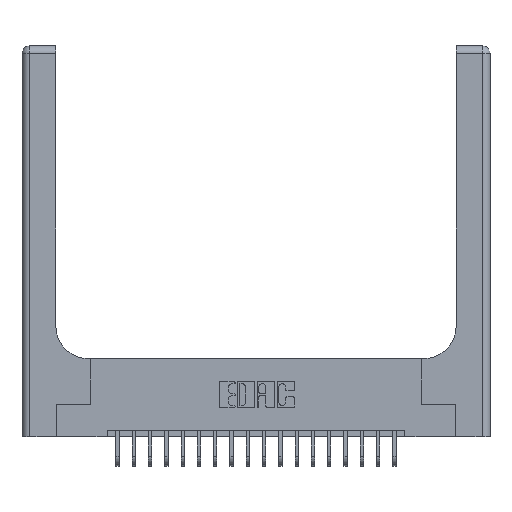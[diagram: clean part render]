
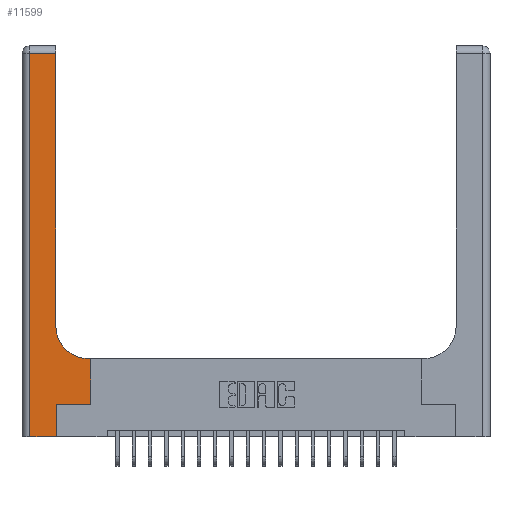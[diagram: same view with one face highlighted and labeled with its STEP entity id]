
A CAD part, top view. The second image highlights one B-rep face of the part: STEP entity #11599.
In plain terms, the highlighted planar face has unit normal (0, 0, 1).
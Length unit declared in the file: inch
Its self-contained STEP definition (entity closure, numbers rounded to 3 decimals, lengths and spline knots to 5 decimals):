
#209 = DIRECTION ( 'NONE',  ( 1., 0., 0. ) ) ;
#285 = CARTESIAN_POINT ( 'NONE',  ( 0.26, 2.94, 0.37 ) ) ;
#312 = LINE ( 'NONE', #4425, #4010 ) ;
#633 = VERTEX_POINT ( 'NONE', #685 ) ;
#685 = CARTESIAN_POINT ( 'NONE',  ( 0.51, 0.6, 0.37 ) ) ;
#1783 = DIRECTION ( 'NONE',  ( -1., 0., 0. ) ) ;
#2127 = VERTEX_POINT ( 'NONE', #19964 ) ;
#2364 = ORIENTED_EDGE ( 'NONE', *, *, #2592, .T. ) ;
#2566 = CARTESIAN_POINT ( 'NONE',  ( 0.06, 2.94, 0.37 ) ) ;
#2592 = EDGE_CURVE ( 'NONE', #12691, #8772, #11009, .T. ) ;
#2869 = CARTESIAN_POINT ( 'NONE',  ( 0.265, 0., 0.37 ) ) ;
#3447 = DIRECTION ( 'NONE',  ( 0., 1., 0. ) ) ;
#3495 = LINE ( 'NONE', #10424, #6220 ) ;
#3815 = ORIENTED_EDGE ( 'NONE', *, *, #8806, .T. ) ;
#4010 = VECTOR ( 'NONE', #4310, 39.37008 ) ;
#4310 = DIRECTION ( 'NONE',  ( 1., 0., 0. ) ) ;
#4425 = CARTESIAN_POINT ( 'NONE',  ( 0.265, 0.25, 0.37 ) ) ;
#4472 = LINE ( 'NONE', #2869, #11944 ) ;
#4580 = CARTESIAN_POINT ( 'NONE',  ( 0.528, 0.25, 0.37 ) ) ;
#4842 = ORIENTED_EDGE ( 'NONE', *, *, #12729, .T. ) ;
#5318 = DIRECTION ( 'NONE',  ( 0., -1., 0. ) ) ;
#5463 = LINE ( 'NONE', #12450, #17801 ) ;
#5824 = VERTEX_POINT ( 'NONE', #20247 ) ;
#6113 = VECTOR ( 'NONE', #5318, 39.37008 ) ;
#6220 = VECTOR ( 'NONE', #1783, 39.37008 ) ;
#7289 = VERTEX_POINT ( 'NONE', #4580 ) ;
#7507 = DIRECTION ( 'NONE',  ( -1., 0., 0. ) ) ;
#7570 = AXIS2_PLACEMENT_3D ( 'NONE', #12461, #14066, #7507 ) ;
#8772 = VERTEX_POINT ( 'NONE', #285 ) ;
#8806 = EDGE_CURVE ( 'NONE', #14880, #15694, #12308, .T. ) ;
#9416 = VECTOR ( 'NONE', #9668, 39.37008 ) ;
#9668 = DIRECTION ( 'NONE',  ( -1., 0., 0. ) ) ;
#10424 = CARTESIAN_POINT ( 'NONE',  ( 0., 2.94, 0.37 ) ) ;
#11009 = LINE ( 'NONE', #19734, #21687 ) ;
#11113 = LINE ( 'NONE', #14728, #9416 ) ;
#11599 = ADVANCED_FACE ( 'NONE', ( #15104 ), #21183, .F. ) ;
#11929 = EDGE_CURVE ( 'NONE', #7289, #18586, #17374, .T. ) ;
#11944 = VECTOR ( 'NONE', #22113, 39.37008 ) ;
#12308 = LINE ( 'NONE', #17417, #6113 ) ;
#12450 = CARTESIAN_POINT ( 'NONE',  ( 0., 0., 0.37 ) ) ;
#12461 = CARTESIAN_POINT ( 'NONE',  ( 0., 3., 0.37 ) ) ;
#12691 = VERTEX_POINT ( 'NONE', #18587 ) ;
#12729 = EDGE_CURVE ( 'NONE', #18586, #633, #11113, .T. ) ;
#12978 = EDGE_CURVE ( 'NONE', #2127, #5824, #4472, .T. ) ;
#13715 = ORIENTED_EDGE ( 'NONE', *, *, #11929, .T. ) ;
#13774 = EDGE_CURVE ( 'NONE', #5824, #7289, #312, .T. ) ;
#14066 = DIRECTION ( 'NONE',  ( 0., 0., -1. ) ) ;
#14306 = ORIENTED_EDGE ( 'NONE', *, *, #15062, .T. ) ;
#14728 = CARTESIAN_POINT ( 'NONE',  ( 0.26, 0.6, 0.37 ) ) ;
#14880 = VERTEX_POINT ( 'NONE', #2566 ) ;
#14966 = CARTESIAN_POINT ( 'NONE',  ( 0.06, 0., 0.37 ) ) ;
#15062 = EDGE_CURVE ( 'NONE', #633, #12691, #16356, .T. ) ;
#15104 = FACE_OUTER_BOUND ( 'NONE', #17996, .T. ) ;
#15547 = DIRECTION ( 'NONE',  ( 0., 0., -1. ) ) ;
#15656 = CARTESIAN_POINT ( 'NONE',  ( 0.528, 0.25, 0.37 ) ) ;
#15694 = VERTEX_POINT ( 'NONE', #14966 ) ;
#16225 = DIRECTION ( 'NONE',  ( 0., 1., 0. ) ) ;
#16356 = CIRCLE ( 'NONE', #17792, 0.25 ) ;
#16542 = CARTESIAN_POINT ( 'NONE',  ( 0.528, 0.6, 0.37 ) ) ;
#17286 = ORIENTED_EDGE ( 'NONE', *, *, #19288, .T. ) ;
#17374 = LINE ( 'NONE', #15656, #18752 ) ;
#17417 = CARTESIAN_POINT ( 'NONE',  ( 0.06, 3., 0.37 ) ) ;
#17784 = EDGE_CURVE ( 'NONE', #8772, #14880, #3495, .T. ) ;
#17792 = AXIS2_PLACEMENT_3D ( 'NONE', #20975, #15547, #19046 ) ;
#17801 = VECTOR ( 'NONE', #209, 39.37008 ) ;
#17996 = EDGE_LOOP ( 'NONE', ( #2364, #21534, #3815, #17286, #18965, #21303, #13715, #4842, #14306 ) ) ;
#18586 = VERTEX_POINT ( 'NONE', #16542 ) ;
#18587 = CARTESIAN_POINT ( 'NONE',  ( 0.26, 0.85, 0.37 ) ) ;
#18752 = VECTOR ( 'NONE', #3447, 39.37008 ) ;
#18965 = ORIENTED_EDGE ( 'NONE', *, *, #12978, .T. ) ;
#19046 = DIRECTION ( 'NONE',  ( 1., 0., 0. ) ) ;
#19288 = EDGE_CURVE ( 'NONE', #15694, #2127, #5463, .T. ) ;
#19734 = CARTESIAN_POINT ( 'NONE',  ( 0.26, 3., 0.37 ) ) ;
#19964 = CARTESIAN_POINT ( 'NONE',  ( 0.265, 0., 0.37 ) ) ;
#20247 = CARTESIAN_POINT ( 'NONE',  ( 0.265, 0.25, 0.37 ) ) ;
#20975 = CARTESIAN_POINT ( 'NONE',  ( 0.51, 0.85, 0.37 ) ) ;
#21183 = PLANE ( 'NONE',  #7570 ) ;
#21303 = ORIENTED_EDGE ( 'NONE', *, *, #13774, .T. ) ;
#21534 = ORIENTED_EDGE ( 'NONE', *, *, #17784, .T. ) ;
#21687 = VECTOR ( 'NONE', #16225, 39.37008 ) ;
#22113 = DIRECTION ( 'NONE',  ( 0., 1., 0. ) ) ;
